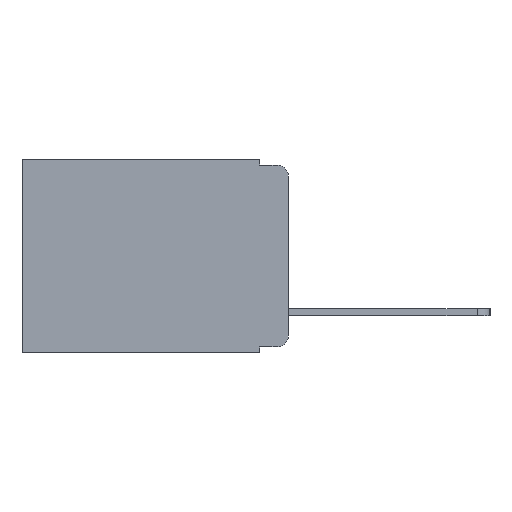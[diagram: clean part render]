
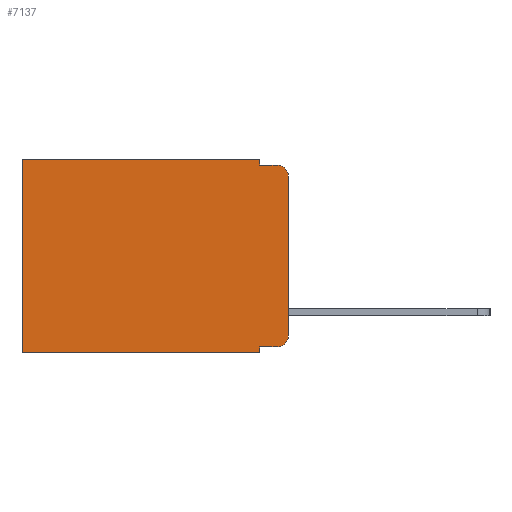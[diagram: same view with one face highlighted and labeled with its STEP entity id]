
A CAD part, left-side view. The second image highlights one B-rep face of the part: STEP entity #7137.
In plain terms, the highlighted planar face has unit normal (-1, 0, 0).
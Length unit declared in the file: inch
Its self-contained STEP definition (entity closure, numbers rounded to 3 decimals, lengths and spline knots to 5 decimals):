
#23 = CARTESIAN_POINT ( 'NONE',  ( 0.298, 0.051, 0. ) ) ;
#87 = VERTEX_POINT ( 'NONE', #14999 ) ;
#94 = VERTEX_POINT ( 'NONE', #4632 ) ;
#160 = CARTESIAN_POINT ( 'NONE',  ( 0.298, 0.02, -0.01 ) ) ;
#207 = AXIS2_PLACEMENT_3D ( 'NONE', #13661, #13549, #7358 ) ;
#247 = VERTEX_POINT ( 'NONE', #5794 ) ;
#621 = DIRECTION ( 'NONE',  ( 0., 0., -1. ) ) ;
#831 = VECTOR ( 'NONE', #11025, 39.37008 ) ;
#965 = LINE ( 'NONE', #10887, #7713 ) ;
#1006 = VERTEX_POINT ( 'NONE', #11224 ) ;
#1031 = CIRCLE ( 'NONE', #15543, 0.02 ) ;
#1093 = ORIENTED_EDGE ( 'NONE', *, *, #5292, .F. ) ;
#1346 = DIRECTION ( 'NONE',  ( 0., 0., -1. ) ) ;
#1739 = VECTOR ( 'NONE', #621, 39.37008 ) ;
#1827 = EDGE_CURVE ( 'NONE', #9857, #247, #13589, .T. ) ;
#1997 = ORIENTED_EDGE ( 'NONE', *, *, #7252, .T. ) ;
#2077 = CARTESIAN_POINT ( 'NONE',  ( 0.298, 0., 0. ) ) ;
#2219 = VERTEX_POINT ( 'NONE', #16424 ) ;
#3789 = VECTOR ( 'NONE', #14595, 39.37008 ) ;
#4252 = VERTEX_POINT ( 'NONE', #160 ) ;
#4530 = EDGE_CURVE ( 'NONE', #1006, #94, #13727, .T. ) ;
#4632 = CARTESIAN_POINT ( 'NONE',  ( 0.298, 0.051, -0.343 ) ) ;
#4668 = VERTEX_POINT ( 'NONE', #6414 ) ;
#4961 = ORIENTED_EDGE ( 'NONE', *, *, #12216, .T. ) ;
#5292 = EDGE_CURVE ( 'NONE', #94, #4668, #965, .T. ) ;
#5544 = CARTESIAN_POINT ( 'NONE',  ( 0.298, 0., -0.03 ) ) ;
#5590 = LINE ( 'NONE', #12087, #12499 ) ;
#5794 = CARTESIAN_POINT ( 'NONE',  ( 0.298, 0.051, -0.01 ) ) ;
#5886 = ORIENTED_EDGE ( 'NONE', *, *, #15582, .F. ) ;
#6414 = CARTESIAN_POINT ( 'NONE',  ( 0.298, 0.473, -0.343 ) ) ;
#6536 = VECTOR ( 'NONE', #11592, 39.37008 ) ;
#6731 = PLANE ( 'NONE',  #11014 ) ;
#7137 = ADVANCED_FACE ( 'NONE', ( #17143 ), #6731, .F. ) ;
#7252 = EDGE_CURVE ( 'NONE', #87, #17005, #15534, .T. ) ;
#7358 = DIRECTION ( 'NONE',  ( 0., 0., -1. ) ) ;
#7556 = LINE ( 'NONE', #13233, #3789 ) ;
#7713 = VECTOR ( 'NONE', #12463, 39.37008 ) ;
#8052 = ORIENTED_EDGE ( 'NONE', *, *, #11983, .F. ) ;
#8895 = LINE ( 'NONE', #16343, #831 ) ;
#9571 = DIRECTION ( 'NONE',  ( 0., 0., -1. ) ) ;
#9614 = VERTEX_POINT ( 'NONE', #5544 ) ;
#9857 = VERTEX_POINT ( 'NONE', #10231 ) ;
#9895 = DIRECTION ( 'NONE',  ( -1., 0., 0. ) ) ;
#10150 = VECTOR ( 'NONE', #17805, 39.37008 ) ;
#10231 = CARTESIAN_POINT ( 'NONE',  ( 0.298, 0.051, 0. ) ) ;
#10242 = ORIENTED_EDGE ( 'NONE', *, *, #17501, .T. ) ;
#10246 = CARTESIAN_POINT ( 'NONE',  ( 0.298, 0.473, 0. ) ) ;
#10549 = EDGE_LOOP ( 'NONE', ( #8052, #4961, #5886, #13602, #10242, #14462, #1093, #16913, #14659, #1997 ) ) ;
#10887 = CARTESIAN_POINT ( 'NONE',  ( 0.298, 0., -0.343 ) ) ;
#11014 = AXIS2_PLACEMENT_3D ( 'NONE', #16098, #15625, #17075 ) ;
#11025 = DIRECTION ( 'NONE',  ( 0., -1., 0. ) ) ;
#11061 = EDGE_CURVE ( 'NONE', #2219, #4668, #17312, .T. ) ;
#11224 = CARTESIAN_POINT ( 'NONE',  ( 0.298, 0.051, -0.333 ) ) ;
#11294 = CARTESIAN_POINT ( 'NONE',  ( 0.298, 0., -0.313 ) ) ;
#11592 = DIRECTION ( 'NONE',  ( 0., 0., -1. ) ) ;
#11905 = CARTESIAN_POINT ( 'NONE',  ( 0.298, 0.051, 0. ) ) ;
#11983 = EDGE_CURVE ( 'NONE', #9614, #17005, #12934, .T. ) ;
#12087 = CARTESIAN_POINT ( 'NONE',  ( 0.298, 0., 0. ) ) ;
#12216 = EDGE_CURVE ( 'NONE', #9614, #4252, #1031, .T. ) ;
#12463 = DIRECTION ( 'NONE',  ( 0., 1., 0. ) ) ;
#12499 = VECTOR ( 'NONE', #13454, 39.37008 ) ;
#12934 = LINE ( 'NONE', #2077, #1739 ) ;
#13167 = VECTOR ( 'NONE', #9571, 39.37008 ) ;
#13233 = CARTESIAN_POINT ( 'NONE',  ( 0.298, 0.051, -0.333 ) ) ;
#13454 = DIRECTION ( 'NONE',  ( 0., 1., 0. ) ) ;
#13549 = DIRECTION ( 'NONE',  ( -1., 0., 0. ) ) ;
#13589 = LINE ( 'NONE', #11905, #13167 ) ;
#13602 = ORIENTED_EDGE ( 'NONE', *, *, #1827, .F. ) ;
#13661 = CARTESIAN_POINT ( 'NONE',  ( 0.298, 0.02, -0.313 ) ) ;
#13727 = LINE ( 'NONE', #23, #10150 ) ;
#14462 = ORIENTED_EDGE ( 'NONE', *, *, #11061, .T. ) ;
#14595 = DIRECTION ( 'NONE',  ( 0., -1., 0. ) ) ;
#14659 = ORIENTED_EDGE ( 'NONE', *, *, #16146, .T. ) ;
#14999 = CARTESIAN_POINT ( 'NONE',  ( 0.298, 0.02, -0.333 ) ) ;
#15534 = CIRCLE ( 'NONE', #207, 0.02 ) ;
#15543 = AXIS2_PLACEMENT_3D ( 'NONE', #17849, #9895, #1346 ) ;
#15582 = EDGE_CURVE ( 'NONE', #247, #4252, #8895, .T. ) ;
#15625 = DIRECTION ( 'NONE',  ( 1., 0., 0. ) ) ;
#16098 = CARTESIAN_POINT ( 'NONE',  ( 0.298, 0., 0. ) ) ;
#16146 = EDGE_CURVE ( 'NONE', #1006, #87, #7556, .T. ) ;
#16343 = CARTESIAN_POINT ( 'NONE',  ( 0.298, 0.051, -0.01 ) ) ;
#16424 = CARTESIAN_POINT ( 'NONE',  ( 0.298, 0.473, 0. ) ) ;
#16913 = ORIENTED_EDGE ( 'NONE', *, *, #4530, .F. ) ;
#17005 = VERTEX_POINT ( 'NONE', #11294 ) ;
#17075 = DIRECTION ( 'NONE',  ( 0., 0., -1. ) ) ;
#17143 = FACE_OUTER_BOUND ( 'NONE', #10549, .T. ) ;
#17312 = LINE ( 'NONE', #10246, #6536 ) ;
#17501 = EDGE_CURVE ( 'NONE', #9857, #2219, #5590, .T. ) ;
#17805 = DIRECTION ( 'NONE',  ( 0., 0., -1. ) ) ;
#17849 = CARTESIAN_POINT ( 'NONE',  ( 0.298, 0.02, -0.03 ) ) ;
